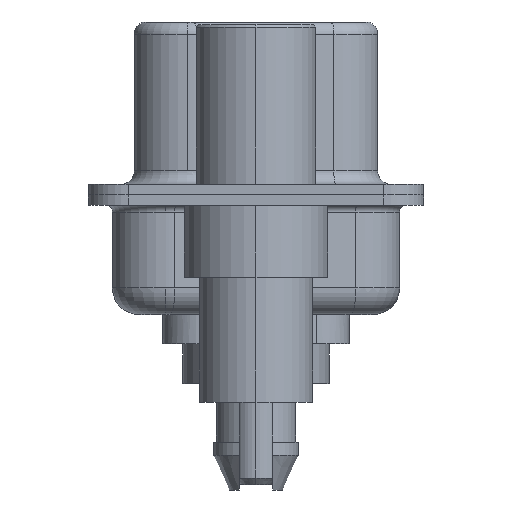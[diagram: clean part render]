
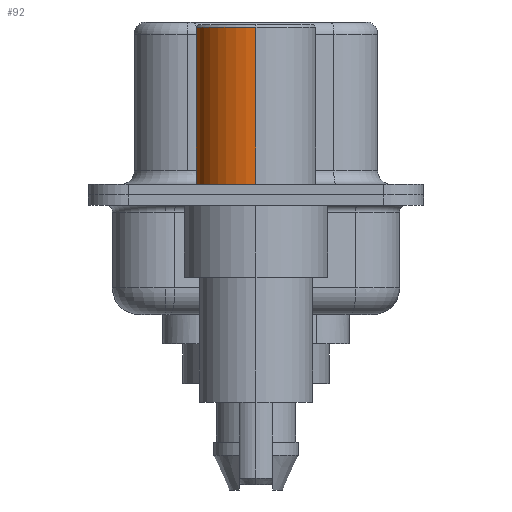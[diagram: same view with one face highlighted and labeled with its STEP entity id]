
A CAD part, left-side view. The second image highlights one B-rep face of the part: STEP entity #92.
In plain terms, the highlighted cylindrical face has radius 2.25 mm (diameter 4.5 mm), a partial arc.
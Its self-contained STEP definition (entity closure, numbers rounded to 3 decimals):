
#92 = ADVANCED_FACE ( 'NONE', ( #14264 ), #7891, .T. ) ;
#480 = ORIENTED_EDGE ( 'NONE', *, *, #5923, .F. ) ;
#734 = DIRECTION ( 'NONE',  ( 1., 0., 0. ) ) ;
#2276 = EDGE_LOOP ( 'NONE', ( #13292, #10786, #5509, #480 ) ) ;
#2575 = AXIS2_PLACEMENT_3D ( 'NONE', #8794, #5374, #5965 ) ;
#2770 = VERTEX_POINT ( 'NONE', #7569 ) ;
#4251 = CARTESIAN_POINT ( 'NONE',  ( -2.25, 0., 6.3 ) ) ;
#4703 = CIRCLE ( 'NONE', #12333, 2.25 ) ;
#4725 = AXIS2_PLACEMENT_3D ( 'NONE', #9195, #10994, #734 ) ;
#5113 = EDGE_CURVE ( 'NONE', #8953, #12012, #4703, .T. ) ;
#5374 = DIRECTION ( 'NONE',  ( 0., 0., 1. ) ) ;
#5442 = EDGE_CURVE ( 'NONE', #10565, #2770, #10706, .T. ) ;
#5509 = ORIENTED_EDGE ( 'NONE', *, *, #5113, .F. ) ;
#5605 = LINE ( 'NONE', #7116, #8295 ) ;
#5830 = EDGE_CURVE ( 'NONE', #2770, #12012, #5605, .T. ) ;
#5923 = EDGE_CURVE ( 'NONE', #10565, #8953, #6842, .T. ) ;
#5965 = DIRECTION ( 'NONE',  ( 1., 0., 0. ) ) ;
#6318 = DIRECTION ( 'NONE',  ( 0., 0., 1. ) ) ;
#6677 = CARTESIAN_POINT ( 'NONE',  ( 2.25, 0., 0.581 ) ) ;
#6686 = DIRECTION ( 'NONE',  ( 0., 0., 1. ) ) ;
#6842 = LINE ( 'NONE', #6677, #9951 ) ;
#7116 = CARTESIAN_POINT ( 'NONE',  ( -2.25, 0., 0.581 ) ) ;
#7569 = CARTESIAN_POINT ( 'NONE',  ( -2.25, 0., 0.4 ) ) ;
#7891 = CYLINDRICAL_SURFACE ( 'NONE', #4725, 2.25 ) ;
#8295 = VECTOR ( 'NONE', #6686, 1000. ) ;
#8512 = DIRECTION ( 'NONE',  ( 1., 0., 0. ) ) ;
#8794 = CARTESIAN_POINT ( 'NONE',  ( 0., 0., 0.4 ) ) ;
#8953 = VERTEX_POINT ( 'NONE', #9445 ) ;
#9195 = CARTESIAN_POINT ( 'NONE',  ( 0., 0., 0.581 ) ) ;
#9445 = CARTESIAN_POINT ( 'NONE',  ( 2.25, 0., 6.3 ) ) ;
#9951 = VECTOR ( 'NONE', #6318, 1000. ) ;
#10565 = VERTEX_POINT ( 'NONE', #11192 ) ;
#10706 = CIRCLE ( 'NONE', #2575, 2.25 ) ;
#10786 = ORIENTED_EDGE ( 'NONE', *, *, #5830, .T. ) ;
#10994 = DIRECTION ( 'NONE',  ( 0., 0., 1. ) ) ;
#11192 = CARTESIAN_POINT ( 'NONE',  ( 2.25, 0., 0.4 ) ) ;
#12012 = VERTEX_POINT ( 'NONE', #4251 ) ;
#12014 = DIRECTION ( 'NONE',  ( 0., 0., 1. ) ) ;
#12069 = CARTESIAN_POINT ( 'NONE',  ( 0., 0., 6.3 ) ) ;
#12333 = AXIS2_PLACEMENT_3D ( 'NONE', #12069, #12014, #8512 ) ;
#13292 = ORIENTED_EDGE ( 'NONE', *, *, #5442, .T. ) ;
#14264 = FACE_OUTER_BOUND ( 'NONE', #2276, .T. ) ;
